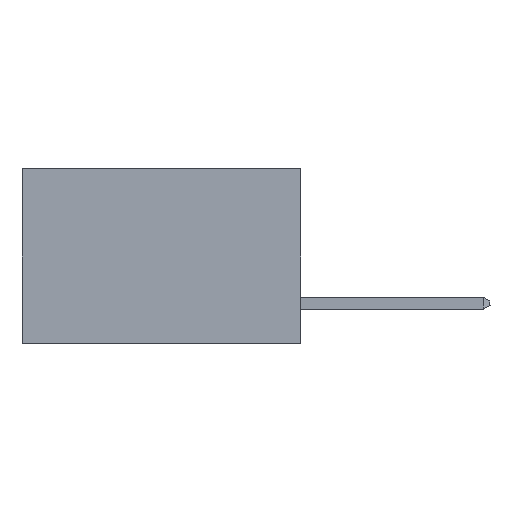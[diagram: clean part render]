
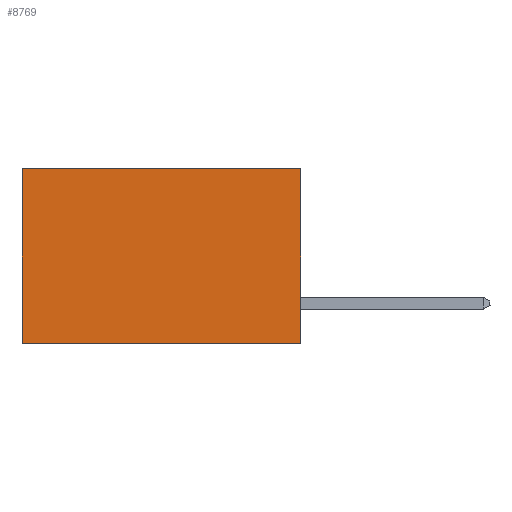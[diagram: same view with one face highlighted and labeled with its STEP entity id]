
A CAD part, left-side view. The second image highlights one B-rep face of the part: STEP entity #8769.
In plain terms, the highlighted planar face has unit normal (-1, 0, 0).
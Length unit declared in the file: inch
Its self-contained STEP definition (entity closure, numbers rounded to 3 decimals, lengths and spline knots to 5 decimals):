
#21 = ORIENTED_EDGE ( 'NONE', *, *, #5266, .T. ) ;
#121 = LINE ( 'NONE', #10363, #8133 ) ;
#660 = FACE_OUTER_BOUND ( 'NONE', #7589, .T. ) ;
#705 = ORIENTED_EDGE ( 'NONE', *, *, #7135, .F. ) ;
#802 = DIRECTION ( 'NONE',  ( 0., 0., -1. ) ) ;
#949 = CARTESIAN_POINT ( 'NONE',  ( 0.277, 0.59, -0.37 ) ) ;
#950 = ORIENTED_EDGE ( 'NONE', *, *, #4233, .F. ) ;
#977 = CARTESIAN_POINT ( 'NONE',  ( 0.277, 0., -0.37 ) ) ;
#1118 = ORIENTED_EDGE ( 'NONE', *, *, #3186, .T. ) ;
#3186 = EDGE_CURVE ( 'NONE', #12252, #6270, #121, .T. ) ;
#3406 = PLANE ( 'NONE',  #9247 ) ;
#4233 = EDGE_CURVE ( 'NONE', #12252, #13136, #9402, .T. ) ;
#4480 = DIRECTION ( 'NONE',  ( 1., 0., 0. ) ) ;
#4646 = CARTESIAN_POINT ( 'NONE',  ( 0.277, 0.59, -0.37 ) ) ;
#4661 = DIRECTION ( 'NONE',  ( 0., 1., 0. ) ) ;
#5266 = EDGE_CURVE ( 'NONE', #6270, #9569, #5752, .T. ) ;
#5752 = LINE ( 'NONE', #949, #7942 ) ;
#5789 = CARTESIAN_POINT ( 'NONE',  ( 0.277, 0.59, 0. ) ) ;
#6270 = VERTEX_POINT ( 'NONE', #5789 ) ;
#6374 = DIRECTION ( 'NONE',  ( 0., 0., -1. ) ) ;
#6650 = VECTOR ( 'NONE', #6374, 39.37008 ) ;
#7077 = CARTESIAN_POINT ( 'NONE',  ( 0.277, 0., -0.37 ) ) ;
#7135 = EDGE_CURVE ( 'NONE', #13136, #9569, #8075, .T. ) ;
#7218 = CARTESIAN_POINT ( 'NONE',  ( 0.277, 0., 0. ) ) ;
#7589 = EDGE_LOOP ( 'NONE', ( #21, #705, #950, #1118 ) ) ;
#7942 = VECTOR ( 'NONE', #802, 39.37008 ) ;
#8075 = LINE ( 'NONE', #9283, #13164 ) ;
#8133 = VECTOR ( 'NONE', #4661, 39.37008 ) ;
#8769 = ADVANCED_FACE ( 'NONE', ( #660 ), #3406, .F. ) ;
#9247 = AXIS2_PLACEMENT_3D ( 'NONE', #10774, #4480, #11797 ) ;
#9283 = CARTESIAN_POINT ( 'NONE',  ( 0.277, 0., -0.37 ) ) ;
#9402 = LINE ( 'NONE', #7077, #6650 ) ;
#9569 = VERTEX_POINT ( 'NONE', #4646 ) ;
#10322 = DIRECTION ( 'NONE',  ( 0., 1., 0. ) ) ;
#10363 = CARTESIAN_POINT ( 'NONE',  ( 0.277, 0., 0. ) ) ;
#10774 = CARTESIAN_POINT ( 'NONE',  ( 0.277, 0., -0.37 ) ) ;
#11797 = DIRECTION ( 'NONE',  ( 0., 0., -1. ) ) ;
#12252 = VERTEX_POINT ( 'NONE', #7218 ) ;
#13136 = VERTEX_POINT ( 'NONE', #977 ) ;
#13164 = VECTOR ( 'NONE', #10322, 39.37008 ) ;
